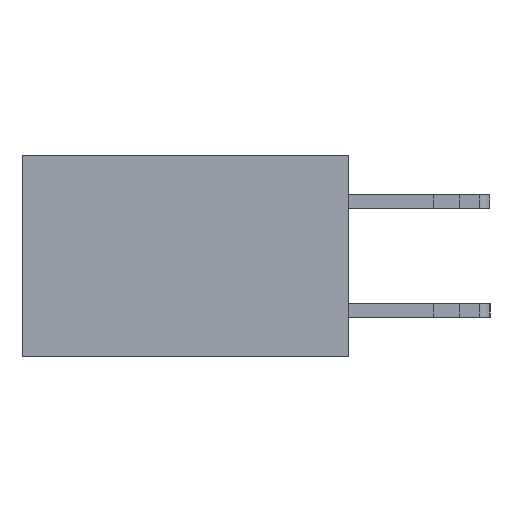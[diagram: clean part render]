
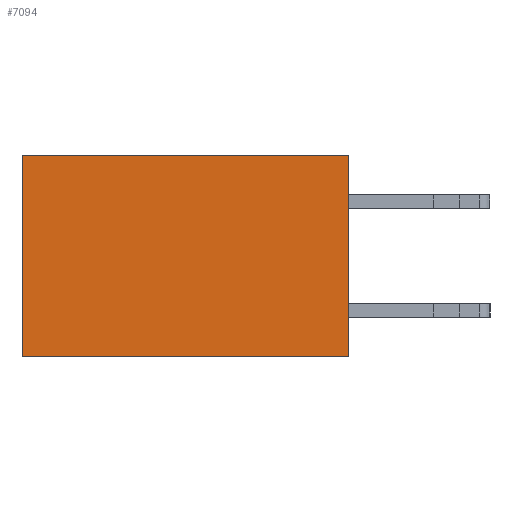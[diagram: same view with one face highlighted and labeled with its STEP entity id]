
A CAD part, left-side view. The second image highlights one B-rep face of the part: STEP entity #7094.
In plain terms, the highlighted planar face has unit normal (-1, 0, 0).
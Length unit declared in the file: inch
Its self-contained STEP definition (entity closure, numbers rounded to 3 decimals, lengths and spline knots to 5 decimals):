
#302 = ORIENTED_EDGE ( 'NONE', *, *, #4484, .T. ) ;
#365 = VERTEX_POINT ( 'NONE', #10623 ) ;
#879 = ORIENTED_EDGE ( 'NONE', *, *, #10886, .F. ) ;
#1483 = DIRECTION ( 'NONE',  ( 1., 0., 0. ) ) ;
#1491 = DIRECTION ( 'NONE',  ( 0., 1., 0. ) ) ;
#2174 = VERTEX_POINT ( 'NONE', #15526 ) ;
#2290 = DIRECTION ( 'NONE',  ( 0., 0., -1. ) ) ;
#2347 = CARTESIAN_POINT ( 'NONE',  ( 0.2615, 0.6, -0.37 ) ) ;
#2782 = CARTESIAN_POINT ( 'NONE',  ( 0.2615, 0., -0.37 ) ) ;
#2856 = VERTEX_POINT ( 'NONE', #4908 ) ;
#3068 = VECTOR ( 'NONE', #6999, 39.37008 ) ;
#3506 = VECTOR ( 'NONE', #1491, 39.37008 ) ;
#4140 = EDGE_LOOP ( 'NONE', ( #302, #5571, #879, #16199 ) ) ;
#4279 = AXIS2_PLACEMENT_3D ( 'NONE', #6937, #1483, #10605 ) ;
#4484 = EDGE_CURVE ( 'NONE', #365, #2174, #15189, .T. ) ;
#4908 = CARTESIAN_POINT ( 'NONE',  ( 0.2615, 0., 0. ) ) ;
#5459 = VECTOR ( 'NONE', #2290, 39.37008 ) ;
#5571 = ORIENTED_EDGE ( 'NONE', *, *, #9658, .F. ) ;
#5626 = CARTESIAN_POINT ( 'NONE',  ( 0.2615, 0., 0. ) ) ;
#6937 = CARTESIAN_POINT ( 'NONE',  ( 0.2615, 0., -0.37 ) ) ;
#6999 = DIRECTION ( 'NONE',  ( 0., 0., -1. ) ) ;
#7094 = ADVANCED_FACE ( 'NONE', ( #7205 ), #9364, .F. ) ;
#7205 = FACE_OUTER_BOUND ( 'NONE', #4140, .T. ) ;
#9364 = PLANE ( 'NONE',  #4279 ) ;
#9404 = DIRECTION ( 'NONE',  ( 0., 1., 0. ) ) ;
#9425 = CARTESIAN_POINT ( 'NONE',  ( 0.2615, 0., -0.37 ) ) ;
#9658 = EDGE_CURVE ( 'NONE', #15164, #2174, #13922, .T. ) ;
#9913 = LINE ( 'NONE', #9425, #3068 ) ;
#10294 = LINE ( 'NONE', #5626, #3506 ) ;
#10605 = DIRECTION ( 'NONE',  ( 0., 0., -1. ) ) ;
#10623 = CARTESIAN_POINT ( 'NONE',  ( 0.2615, 0.6, 0. ) ) ;
#10846 = EDGE_CURVE ( 'NONE', #2856, #365, #10294, .T. ) ;
#10886 = EDGE_CURVE ( 'NONE', #2856, #15164, #9913, .T. ) ;
#11890 = CARTESIAN_POINT ( 'NONE',  ( 0.2615, 0., -0.37 ) ) ;
#13922 = LINE ( 'NONE', #11890, #16290 ) ;
#15164 = VERTEX_POINT ( 'NONE', #2782 ) ;
#15189 = LINE ( 'NONE', #2347, #5459 ) ;
#15526 = CARTESIAN_POINT ( 'NONE',  ( 0.2615, 0.6, -0.37 ) ) ;
#16199 = ORIENTED_EDGE ( 'NONE', *, *, #10846, .T. ) ;
#16290 = VECTOR ( 'NONE', #9404, 39.37008 ) ;
